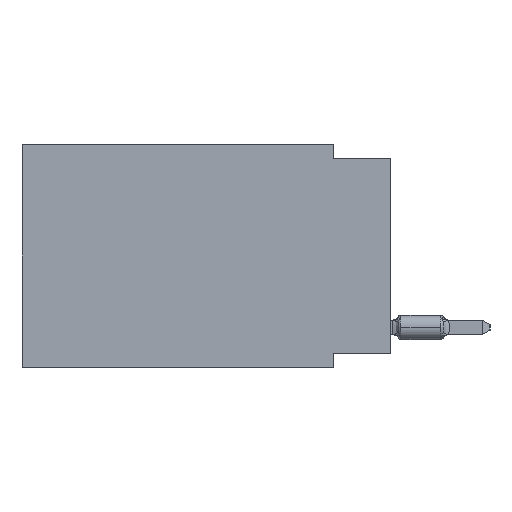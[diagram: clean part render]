
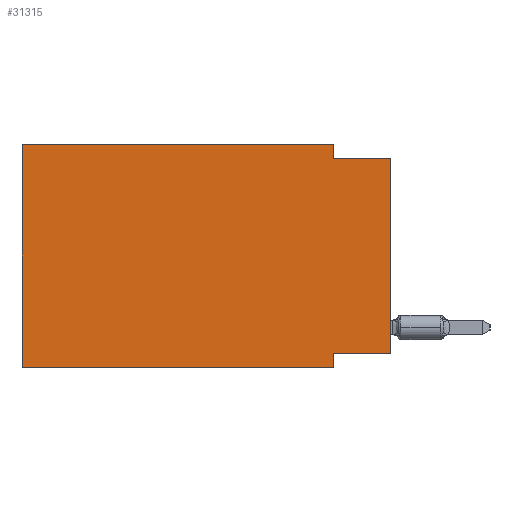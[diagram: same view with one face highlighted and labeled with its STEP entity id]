
A CAD part, left-side view. The second image highlights one B-rep face of the part: STEP entity #31315.
In plain terms, the highlighted planar face has unit normal (-1, 0, 0).
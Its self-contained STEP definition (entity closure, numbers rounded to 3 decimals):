
#2620 = EDGE_CURVE ( 'NONE', #54343, #22556, #60025, .T. ) ;
#2840 = DIRECTION ( 'NONE',  ( 0., 0., 1. ) ) ;
#2913 = CARTESIAN_POINT ( 'NONE',  ( 0., 16.383, 0. ) ) ;
#3336 = LINE ( 'NONE', #26686, #50804 ) ;
#6630 = CARTESIAN_POINT ( 'NONE',  ( 0., 2.54, -0.635 ) ) ;
#6989 = VECTOR ( 'NONE', #9333, 1000. ) ;
#9333 = DIRECTION ( 'NONE',  ( 0., 1., 0. ) ) ;
#10031 = DIRECTION ( 'NONE',  ( 0., -1., 0. ) ) ;
#10986 = DIRECTION ( 'NONE',  ( 0., 0., -1. ) ) ;
#11163 = VERTEX_POINT ( 'NONE', #70779 ) ;
#11333 = LINE ( 'NONE', #62300, #46769 ) ;
#12662 = EDGE_CURVE ( 'NONE', #57762, #63497, #40058, .T. ) ;
#13417 = ORIENTED_EDGE ( 'NONE', *, *, #12662, .F. ) ;
#14384 = EDGE_CURVE ( 'NONE', #70486, #62005, #3336, .T. ) ;
#16154 = LINE ( 'NONE', #44898, #59346 ) ;
#18756 = VECTOR ( 'NONE', #63422, 1000. ) ;
#18883 = CARTESIAN_POINT ( 'NONE',  ( 0., 16.383, 0. ) ) ;
#21177 = CARTESIAN_POINT ( 'NONE',  ( 0., 16.383, -9.906 ) ) ;
#22380 = ORIENTED_EDGE ( 'NONE', *, *, #14384, .F. ) ;
#22556 = VERTEX_POINT ( 'NONE', #6630 ) ;
#23350 = CARTESIAN_POINT ( 'NONE',  ( 0., 2.54, 0. ) ) ;
#24156 = ORIENTED_EDGE ( 'NONE', *, *, #44222, .F. ) ;
#24289 = CARTESIAN_POINT ( 'NONE',  ( 0., 2.54, -9.906 ) ) ;
#24986 = DIRECTION ( 'NONE',  ( 1., 0., 0. ) ) ;
#25257 = VECTOR ( 'NONE', #2840, 1000. ) ;
#26686 = CARTESIAN_POINT ( 'NONE',  ( 0., 2.54, -9.906 ) ) ;
#27348 = DIRECTION ( 'NONE',  ( 0., -1., 0. ) ) ;
#28708 = DIRECTION ( 'NONE',  ( 0., 0., -1. ) ) ;
#28931 = CARTESIAN_POINT ( 'NONE',  ( 0., 16.383, 0. ) ) ;
#29947 = EDGE_CURVE ( 'NONE', #22556, #11163, #16154, .T. ) ;
#31229 = ORIENTED_EDGE ( 'NONE', *, *, #50120, .T. ) ;
#31315 = ADVANCED_FACE ( 'NONE', ( #71398 ), #44060, .F. ) ;
#31573 = LINE ( 'NONE', #38456, #25257 ) ;
#32405 = AXIS2_PLACEMENT_3D ( 'NONE', #18883, #24986, #44436 ) ;
#37044 = ORIENTED_EDGE ( 'NONE', *, *, #46166, .T. ) ;
#37609 = CARTESIAN_POINT ( 'NONE',  ( 0., 2.54, 0. ) ) ;
#38440 = LINE ( 'NONE', #56065, #6989 ) ;
#38456 = CARTESIAN_POINT ( 'NONE',  ( 0., 0., 0. ) ) ;
#38803 = EDGE_LOOP ( 'NONE', ( #37044, #61276, #59634, #24156, #13417, #31229, #22380, #74235 ) ) ;
#40058 = LINE ( 'NONE', #28931, #18756 ) ;
#44060 = PLANE ( 'NONE',  #32405 ) ;
#44222 = EDGE_CURVE ( 'NONE', #63497, #54343, #67238, .T. ) ;
#44436 = DIRECTION ( 'NONE',  ( 0., 0., -1. ) ) ;
#44898 = CARTESIAN_POINT ( 'NONE',  ( 0., 0., -0.635 ) ) ;
#46166 = EDGE_CURVE ( 'NONE', #70220, #11163, #31573, .T. ) ;
#46769 = VECTOR ( 'NONE', #69957, 1000. ) ;
#48831 = CARTESIAN_POINT ( 'NONE',  ( 0., 0., -9.271 ) ) ;
#50120 = EDGE_CURVE ( 'NONE', #57762, #62005, #11333, .T. ) ;
#50804 = VECTOR ( 'NONE', #10986, 1000. ) ;
#52144 = CARTESIAN_POINT ( 'NONE',  ( 0., 2.54, -9.271 ) ) ;
#54343 = VERTEX_POINT ( 'NONE', #37609 ) ;
#56065 = CARTESIAN_POINT ( 'NONE',  ( 0., 0., -9.271 ) ) ;
#56113 = CARTESIAN_POINT ( 'NONE',  ( 0., 16.383, 0. ) ) ;
#57716 = EDGE_CURVE ( 'NONE', #70220, #70486, #38440, .T. ) ;
#57762 = VERTEX_POINT ( 'NONE', #21177 ) ;
#59346 = VECTOR ( 'NONE', #10031, 1000. ) ;
#59634 = ORIENTED_EDGE ( 'NONE', *, *, #2620, .F. ) ;
#60025 = LINE ( 'NONE', #23350, #68338 ) ;
#61276 = ORIENTED_EDGE ( 'NONE', *, *, #29947, .F. ) ;
#62005 = VERTEX_POINT ( 'NONE', #24289 ) ;
#62300 = CARTESIAN_POINT ( 'NONE',  ( 0., 16.383, -9.906 ) ) ;
#63422 = DIRECTION ( 'NONE',  ( 0., 0., 1. ) ) ;
#63497 = VERTEX_POINT ( 'NONE', #2913 ) ;
#66807 = VECTOR ( 'NONE', #27348, 1000. ) ;
#67238 = LINE ( 'NONE', #56113, #66807 ) ;
#68338 = VECTOR ( 'NONE', #28708, 1000. ) ;
#69957 = DIRECTION ( 'NONE',  ( 0., -1., 0. ) ) ;
#70220 = VERTEX_POINT ( 'NONE', #48831 ) ;
#70486 = VERTEX_POINT ( 'NONE', #52144 ) ;
#70779 = CARTESIAN_POINT ( 'NONE',  ( 0., 0., -0.635 ) ) ;
#71398 = FACE_OUTER_BOUND ( 'NONE', #38803, .T. ) ;
#74235 = ORIENTED_EDGE ( 'NONE', *, *, #57716, .F. ) ;
